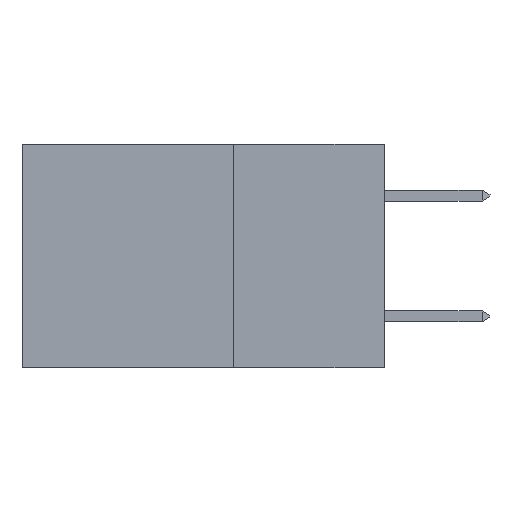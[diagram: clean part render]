
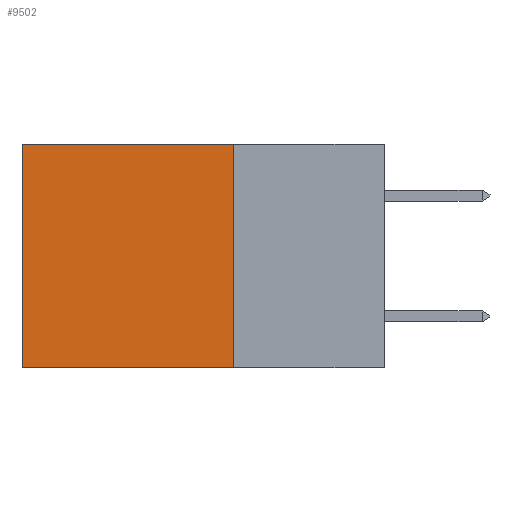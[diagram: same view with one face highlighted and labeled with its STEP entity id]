
A CAD part, left-side view. The second image highlights one B-rep face of the part: STEP entity #9502.
In plain terms, the highlighted planar face has unit normal (-1, 0, 0).
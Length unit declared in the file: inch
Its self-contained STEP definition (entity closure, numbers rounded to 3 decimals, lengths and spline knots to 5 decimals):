
#668 = AXIS2_PLACEMENT_3D ( 'NONE', #16196, #20267, #8316 ) ;
#901 = VECTOR ( 'NONE', #23676, 39.37008 ) ;
#2649 = EDGE_CURVE ( 'NONE', #25032, #22280, #25572, .T. ) ;
#3050 = DIRECTION ( 'NONE',  ( 0., 0., -1. ) ) ;
#3574 = ORIENTED_EDGE ( 'NONE', *, *, #2649, .F. ) ;
#3797 = LINE ( 'NONE', #10802, #14374 ) ;
#3988 = FACE_OUTER_BOUND ( 'NONE', #19114, .T. ) ;
#4338 = VECTOR ( 'NONE', #6966, 39.37008 ) ;
#6204 = LINE ( 'NONE', #17575, #901 ) ;
#6966 = DIRECTION ( 'NONE',  ( 0., 0., -1. ) ) ;
#7044 = VERTEX_POINT ( 'NONE', #19642 ) ;
#7537 = EDGE_CURVE ( 'NONE', #9265, #7044, #13767, .T. ) ;
#8316 = DIRECTION ( 'NONE',  ( 0., 0., -1. ) ) ;
#9265 = VERTEX_POINT ( 'NONE', #23615 ) ;
#9502 = ADVANCED_FACE ( 'NONE', ( #3988 ), #18192, .F. ) ;
#10802 = CARTESIAN_POINT ( 'NONE',  ( 0.2875, 0.25, 0. ) ) ;
#12804 = DIRECTION ( 'NONE',  ( 0., 1., 0. ) ) ;
#13685 = EDGE_CURVE ( 'NONE', #25032, #9265, #3797, .T. ) ;
#13767 = LINE ( 'NONE', #14959, #19054 ) ;
#14353 = CARTESIAN_POINT ( 'NONE',  ( 0.2875, 0.25, 0. ) ) ;
#14374 = VECTOR ( 'NONE', #12804, 39.37008 ) ;
#14959 = CARTESIAN_POINT ( 'NONE',  ( 0.2875, 0.6, 0. ) ) ;
#15754 = CARTESIAN_POINT ( 'NONE',  ( 0.2875, 0.25, -0.37 ) ) ;
#16196 = CARTESIAN_POINT ( 'NONE',  ( 0.2875, 0.25, 0. ) ) ;
#17575 = CARTESIAN_POINT ( 'NONE',  ( 0.2875, 0.25, -0.37 ) ) ;
#18192 = PLANE ( 'NONE',  #668 ) ;
#19054 = VECTOR ( 'NONE', #3050, 39.37008 ) ;
#19069 = ORIENTED_EDGE ( 'NONE', *, *, #22870, .F. ) ;
#19114 = EDGE_LOOP ( 'NONE', ( #24915, #19069, #3574, #23482 ) ) ;
#19642 = CARTESIAN_POINT ( 'NONE',  ( 0.2875, 0.6, -0.37 ) ) ;
#20267 = DIRECTION ( 'NONE',  ( 1., 0., 0. ) ) ;
#22280 = VERTEX_POINT ( 'NONE', #15754 ) ;
#22855 = CARTESIAN_POINT ( 'NONE',  ( 0.2875, 0.25, 0. ) ) ;
#22870 = EDGE_CURVE ( 'NONE', #22280, #7044, #6204, .T. ) ;
#23482 = ORIENTED_EDGE ( 'NONE', *, *, #13685, .T. ) ;
#23615 = CARTESIAN_POINT ( 'NONE',  ( 0.2875, 0.6, 0. ) ) ;
#23676 = DIRECTION ( 'NONE',  ( 0., 1., 0. ) ) ;
#24915 = ORIENTED_EDGE ( 'NONE', *, *, #7537, .T. ) ;
#25032 = VERTEX_POINT ( 'NONE', #14353 ) ;
#25572 = LINE ( 'NONE', #22855, #4338 ) ;
